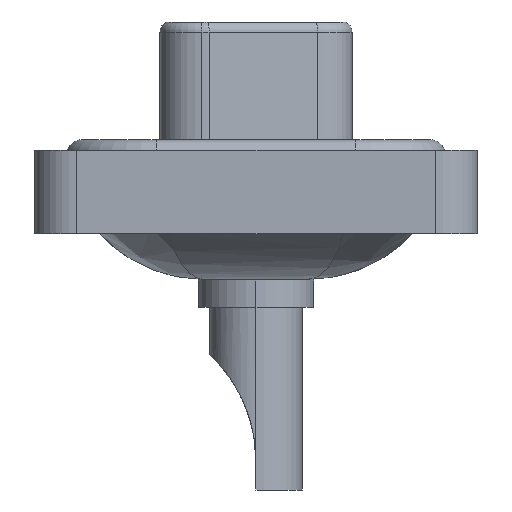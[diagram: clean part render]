
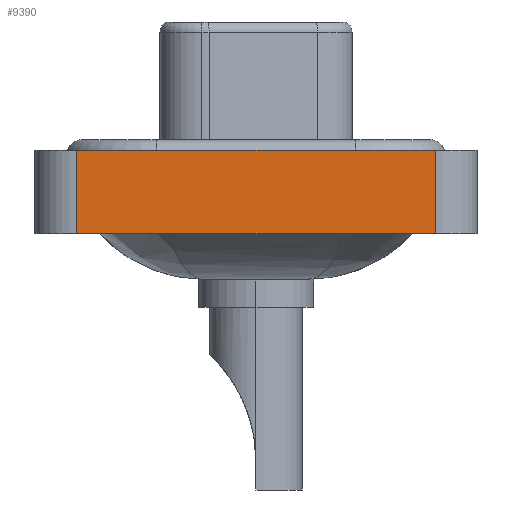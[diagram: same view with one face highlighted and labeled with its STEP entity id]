
A CAD part, left-side view. The second image highlights one B-rep face of the part: STEP entity #9390.
In plain terms, the highlighted planar face has unit normal (-1, 0, 0).
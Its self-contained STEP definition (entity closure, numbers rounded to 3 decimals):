
#224 = DIRECTION ( 'NONE',  ( 0., 0., 1. ) ) ;
#557 = PLANE ( 'NONE',  #11502 ) ;
#1464 = VERTEX_POINT ( 'NONE', #11963 ) ;
#1697 = LINE ( 'NONE', #11334, #13368 ) ;
#1765 = LINE ( 'NONE', #2043, #10682 ) ;
#2043 = CARTESIAN_POINT ( 'NONE',  ( -7.25, -8.55, 0.4 ) ) ;
#2901 = ORIENTED_EDGE ( 'NONE', *, *, #9064, .F. ) ;
#2966 = LINE ( 'NONE', #11062, #16608 ) ;
#4414 = VERTEX_POINT ( 'NONE', #8308 ) ;
#4494 = FACE_OUTER_BOUND ( 'NONE', #11991, .T. ) ;
#4604 = DIRECTION ( 'NONE',  ( 0., -1., 0. ) ) ;
#7323 = DIRECTION ( 'NONE',  ( 0., 0., 1. ) ) ;
#7925 = ORIENTED_EDGE ( 'NONE', *, *, #8484, .F. ) ;
#8308 = CARTESIAN_POINT ( 'NONE',  ( -7.25, 8.55, 0.4 ) ) ;
#8450 = ORIENTED_EDGE ( 'NONE', *, *, #9964, .T. ) ;
#8484 = EDGE_CURVE ( 'NONE', #12740, #4414, #1697, .T. ) ;
#8717 = LINE ( 'NONE', #17424, #17295 ) ;
#9064 = EDGE_CURVE ( 'NONE', #4414, #13686, #1765, .T. ) ;
#9390 = ADVANCED_FACE ( 'NONE', ( #4494 ), #557, .T. ) ;
#9964 = EDGE_CURVE ( 'NONE', #12740, #1464, #8717, .T. ) ;
#10682 = VECTOR ( 'NONE', #11580, 1000. ) ;
#11062 = CARTESIAN_POINT ( 'NONE',  ( -7.25, -8.55, -3.6 ) ) ;
#11334 = CARTESIAN_POINT ( 'NONE',  ( -7.25, 8.55, -3.6 ) ) ;
#11427 = DIRECTION ( 'NONE',  ( 0., 0., 1. ) ) ;
#11502 = AXIS2_PLACEMENT_3D ( 'NONE', #14313, #11563, #7323 ) ;
#11563 = DIRECTION ( 'NONE',  ( -1., 0., 0. ) ) ;
#11580 = DIRECTION ( 'NONE',  ( 0., -1., 0. ) ) ;
#11963 = CARTESIAN_POINT ( 'NONE',  ( -7.25, -8.55, -3.6 ) ) ;
#11991 = EDGE_LOOP ( 'NONE', ( #17519, #2901, #7925, #8450 ) ) ;
#12740 = VERTEX_POINT ( 'NONE', #13331 ) ;
#13331 = CARTESIAN_POINT ( 'NONE',  ( -7.25, 8.55, -3.6 ) ) ;
#13368 = VECTOR ( 'NONE', #224, 1000. ) ;
#13686 = VERTEX_POINT ( 'NONE', #14560 ) ;
#13972 = EDGE_CURVE ( 'NONE', #1464, #13686, #2966, .T. ) ;
#14313 = CARTESIAN_POINT ( 'NONE',  ( -7.25, -8.55, -3.6 ) ) ;
#14560 = CARTESIAN_POINT ( 'NONE',  ( -7.25, -8.55, 0.4 ) ) ;
#16608 = VECTOR ( 'NONE', #11427, 1000. ) ;
#17295 = VECTOR ( 'NONE', #4604, 1000. ) ;
#17424 = CARTESIAN_POINT ( 'NONE',  ( -7.25, -8.55, -3.6 ) ) ;
#17519 = ORIENTED_EDGE ( 'NONE', *, *, #13972, .T. ) ;
